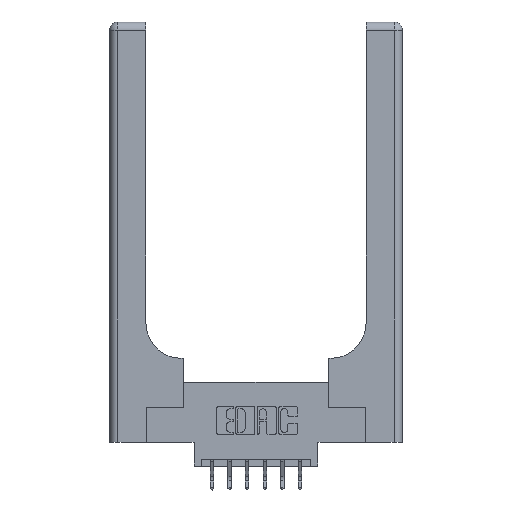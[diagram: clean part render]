
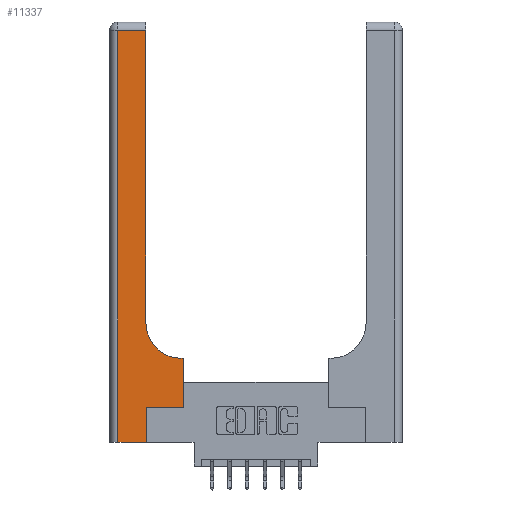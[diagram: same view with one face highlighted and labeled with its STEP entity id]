
A CAD part, top view. The second image highlights one B-rep face of the part: STEP entity #11337.
In plain terms, the highlighted planar face has unit normal (0, 0, 1).
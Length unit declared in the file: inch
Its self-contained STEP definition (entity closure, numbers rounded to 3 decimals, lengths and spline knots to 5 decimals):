
#239 = EDGE_CURVE ( 'NONE', #3046, #4640, #12476, .T. ) ;
#378 = CARTESIAN_POINT ( 'NONE',  ( 0.26, 2.94, 0.37 ) ) ;
#417 = CARTESIAN_POINT ( 'NONE',  ( 0.528, 0.6, 0.37 ) ) ;
#455 = VERTEX_POINT ( 'NONE', #772 ) ;
#557 = LINE ( 'NONE', #7207, #11960 ) ;
#687 = VECTOR ( 'NONE', #8679, 39.37008 ) ;
#772 = CARTESIAN_POINT ( 'NONE',  ( 0.528, 0.25, 0.37 ) ) ;
#989 = VERTEX_POINT ( 'NONE', #12872 ) ;
#1498 = DIRECTION ( 'NONE',  ( 0., 1., 0. ) ) ;
#2483 = VECTOR ( 'NONE', #9329, 39.37008 ) ;
#2563 = CARTESIAN_POINT ( 'NONE',  ( 0.265, 0., 0.37 ) ) ;
#2722 = CARTESIAN_POINT ( 'NONE',  ( 0., 3., 0.37 ) ) ;
#2853 = VERTEX_POINT ( 'NONE', #417 ) ;
#3044 = CARTESIAN_POINT ( 'NONE',  ( 0.06, 0., 0.37 ) ) ;
#3046 = VERTEX_POINT ( 'NONE', #3044 ) ;
#3099 = EDGE_CURVE ( 'NONE', #455, #2853, #3628, .T. ) ;
#3628 = LINE ( 'NONE', #5351, #687 ) ;
#3818 = PLANE ( 'NONE',  #7669 ) ;
#3988 = DIRECTION ( 'NONE',  ( 0., 0., -1. ) ) ;
#4015 = VERTEX_POINT ( 'NONE', #378 ) ;
#4107 = DIRECTION ( 'NONE',  ( 0., -1., 0. ) ) ;
#4640 = VERTEX_POINT ( 'NONE', #2563 ) ;
#4713 = LINE ( 'NONE', #5152, #13161 ) ;
#4844 = CARTESIAN_POINT ( 'NONE',  ( 0.26, 3., 0.37 ) ) ;
#4946 = DIRECTION ( 'NONE',  ( 0., 0., -1. ) ) ;
#5116 = CARTESIAN_POINT ( 'NONE',  ( 0.26, 0.85, 0.37 ) ) ;
#5152 = CARTESIAN_POINT ( 'NONE',  ( 0.265, 0.25, 0.37 ) ) ;
#5309 = ORIENTED_EDGE ( 'NONE', *, *, #14085, .T. ) ;
#5351 = CARTESIAN_POINT ( 'NONE',  ( 0.528, 0.25, 0.37 ) ) ;
#5681 = LINE ( 'NONE', #4844, #8623 ) ;
#5961 = ORIENTED_EDGE ( 'NONE', *, *, #3099, .T. ) ;
#6012 = ORIENTED_EDGE ( 'NONE', *, *, #9111, .T. ) ;
#6141 = VERTEX_POINT ( 'NONE', #13429 ) ;
#6211 = DIRECTION ( 'NONE',  ( -1., 0., 0. ) ) ;
#6614 = VECTOR ( 'NONE', #6916, 39.37008 ) ;
#6764 = EDGE_CURVE ( 'NONE', #4015, #6141, #14198, .T. ) ;
#6916 = DIRECTION ( 'NONE',  ( 1., 0., 0. ) ) ;
#7100 = CARTESIAN_POINT ( 'NONE',  ( 0., 2.94, 0.37 ) ) ;
#7207 = CARTESIAN_POINT ( 'NONE',  ( 0.265, 0., 0.37 ) ) ;
#7669 = AXIS2_PLACEMENT_3D ( 'NONE', #2722, #4946, #12646 ) ;
#7958 = LINE ( 'NONE', #9602, #10208 ) ;
#7986 = VECTOR ( 'NONE', #6211, 39.37008 ) ;
#8007 = EDGE_CURVE ( 'NONE', #2853, #8443, #10915, .T. ) ;
#8079 = EDGE_CURVE ( 'NONE', #989, #455, #4713, .T. ) ;
#8175 = ORIENTED_EDGE ( 'NONE', *, *, #6764, .T. ) ;
#8234 = ORIENTED_EDGE ( 'NONE', *, *, #13542, .T. ) ;
#8246 = ORIENTED_EDGE ( 'NONE', *, *, #8007, .T. ) ;
#8389 = CARTESIAN_POINT ( 'NONE',  ( 0.26, 0.6, 0.37 ) ) ;
#8443 = VERTEX_POINT ( 'NONE', #11395 ) ;
#8623 = VECTOR ( 'NONE', #1498, 39.37008 ) ;
#8679 = DIRECTION ( 'NONE',  ( 0., 1., 0. ) ) ;
#9111 = EDGE_CURVE ( 'NONE', #6141, #3046, #7958, .T. ) ;
#9324 = EDGE_LOOP ( 'NONE', ( #5309, #8175, #6012, #11360, #10463, #12155, #5961, #8246, #8234 ) ) ;
#9329 = DIRECTION ( 'NONE',  ( -1., 0., 0. ) ) ;
#9602 = CARTESIAN_POINT ( 'NONE',  ( 0.06, 3., 0.37 ) ) ;
#10208 = VECTOR ( 'NONE', #4107, 39.37008 ) ;
#10463 = ORIENTED_EDGE ( 'NONE', *, *, #10857, .T. ) ;
#10600 = CARTESIAN_POINT ( 'NONE',  ( 0.51, 0.85, 0.37 ) ) ;
#10857 = EDGE_CURVE ( 'NONE', #4640, #989, #557, .T. ) ;
#10915 = LINE ( 'NONE', #8389, #7986 ) ;
#11337 = ADVANCED_FACE ( 'NONE', ( #11949 ), #3818, .F. ) ;
#11360 = ORIENTED_EDGE ( 'NONE', *, *, #239, .T. ) ;
#11395 = CARTESIAN_POINT ( 'NONE',  ( 0.51, 0.6, 0.37 ) ) ;
#11655 = DIRECTION ( 'NONE',  ( 0., 1., 0. ) ) ;
#11710 = DIRECTION ( 'NONE',  ( 1., 0., 0. ) ) ;
#11949 = FACE_OUTER_BOUND ( 'NONE', #9324, .T. ) ;
#11960 = VECTOR ( 'NONE', #11655, 39.37008 ) ;
#12053 = VERTEX_POINT ( 'NONE', #5116 ) ;
#12155 = ORIENTED_EDGE ( 'NONE', *, *, #8079, .T. ) ;
#12476 = LINE ( 'NONE', #13515, #6614 ) ;
#12646 = DIRECTION ( 'NONE',  ( -1., 0., 0. ) ) ;
#12872 = CARTESIAN_POINT ( 'NONE',  ( 0.265, 0.25, 0.37 ) ) ;
#12873 = AXIS2_PLACEMENT_3D ( 'NONE', #10600, #3988, #11710 ) ;
#12909 = DIRECTION ( 'NONE',  ( 1., 0., 0. ) ) ;
#13161 = VECTOR ( 'NONE', #12909, 39.37008 ) ;
#13297 = CIRCLE ( 'NONE', #12873, 0.25 ) ;
#13429 = CARTESIAN_POINT ( 'NONE',  ( 0.06, 2.94, 0.37 ) ) ;
#13515 = CARTESIAN_POINT ( 'NONE',  ( 0., 0., 0.37 ) ) ;
#13542 = EDGE_CURVE ( 'NONE', #8443, #12053, #13297, .T. ) ;
#14085 = EDGE_CURVE ( 'NONE', #12053, #4015, #5681, .T. ) ;
#14198 = LINE ( 'NONE', #7100, #2483 ) ;
